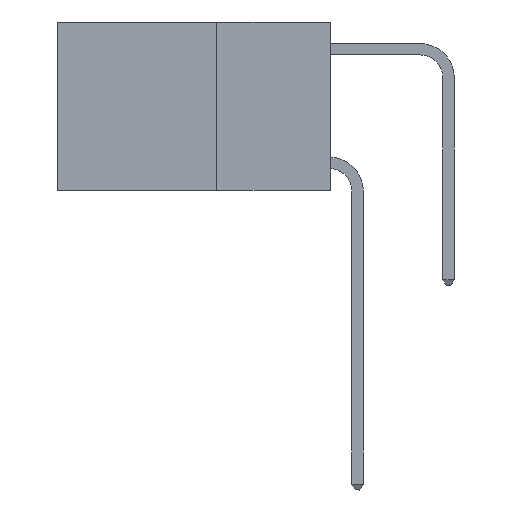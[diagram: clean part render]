
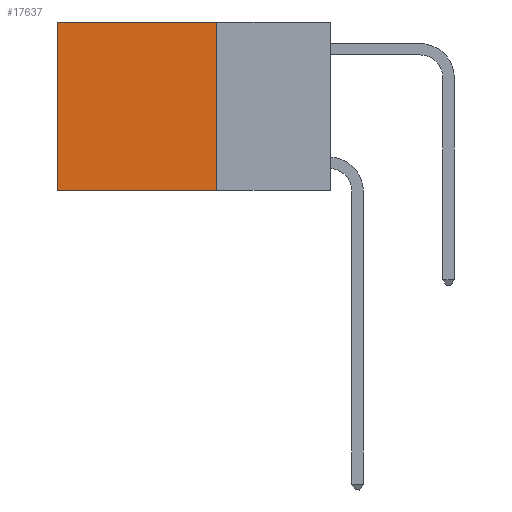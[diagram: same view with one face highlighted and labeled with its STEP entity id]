
A CAD part, left-side view. The second image highlights one B-rep face of the part: STEP entity #17637.
In plain terms, the highlighted planar face has unit normal (-1, 0, 0).
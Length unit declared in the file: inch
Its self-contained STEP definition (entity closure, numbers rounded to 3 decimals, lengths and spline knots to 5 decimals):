
#320 = ORIENTED_EDGE ( 'NONE', *, *, #20586, .F. ) ;
#1253 = CARTESIAN_POINT ( 'NONE',  ( 0.2625, 0.6, 0. ) ) ;
#2351 = AXIS2_PLACEMENT_3D ( 'NONE', #25943, #19576, #7491 ) ;
#5475 = ORIENTED_EDGE ( 'NONE', *, *, #19314, .T. ) ;
#5598 = ORIENTED_EDGE ( 'NONE', *, *, #20037, .F. ) ;
#6199 = VECTOR ( 'NONE', #19068, 39.37008 ) ;
#6403 = CARTESIAN_POINT ( 'NONE',  ( 0.2625, 0.25, 0. ) ) ;
#6913 = VERTEX_POINT ( 'NONE', #6403 ) ;
#7078 = VERTEX_POINT ( 'NONE', #18467 ) ;
#7491 = DIRECTION ( 'NONE',  ( 0., 0., -1. ) ) ;
#7664 = DIRECTION ( 'NONE',  ( 0., 0., -1. ) ) ;
#8567 = DIRECTION ( 'NONE',  ( 0., 1., 0. ) ) ;
#11240 = LINE ( 'NONE', #18738, #12729 ) ;
#11598 = PLANE ( 'NONE',  #2351 ) ;
#12692 = VECTOR ( 'NONE', #8567, 39.37008 ) ;
#12729 = VECTOR ( 'NONE', #25596, 39.37008 ) ;
#13668 = CARTESIAN_POINT ( 'NONE',  ( 0.2625, 0.25, -0.37 ) ) ;
#17259 = EDGE_LOOP ( 'NONE', ( #25081, #5598, #320, #5475 ) ) ;
#17589 = LINE ( 'NONE', #1253, #25044 ) ;
#17637 = ADVANCED_FACE ( 'NONE', ( #19714 ), #11598, .F. ) ;
#18467 = CARTESIAN_POINT ( 'NONE',  ( 0.2625, 0.6, -0.37 ) ) ;
#18738 = CARTESIAN_POINT ( 'NONE',  ( 0.2625, 0.25, -0.37 ) ) ;
#19068 = DIRECTION ( 'NONE',  ( 0., 0., -1. ) ) ;
#19282 = CARTESIAN_POINT ( 'NONE',  ( 0.2625, 0.25, 0. ) ) ;
#19314 = EDGE_CURVE ( 'NONE', #6913, #21622, #21300, .T. ) ;
#19334 = LINE ( 'NONE', #21101, #6199 ) ;
#19576 = DIRECTION ( 'NONE',  ( 1., 0., 0. ) ) ;
#19714 = FACE_OUTER_BOUND ( 'NONE', #17259, .T. ) ;
#20037 = EDGE_CURVE ( 'NONE', #26081, #7078, #11240, .T. ) ;
#20586 = EDGE_CURVE ( 'NONE', #6913, #26081, #19334, .T. ) ;
#21101 = CARTESIAN_POINT ( 'NONE',  ( 0.2625, 0.25, 0. ) ) ;
#21300 = LINE ( 'NONE', #19282, #12692 ) ;
#21622 = VERTEX_POINT ( 'NONE', #26560 ) ;
#25044 = VECTOR ( 'NONE', #7664, 39.37008 ) ;
#25081 = ORIENTED_EDGE ( 'NONE', *, *, #26074, .T. ) ;
#25596 = DIRECTION ( 'NONE',  ( 0., 1., 0. ) ) ;
#25943 = CARTESIAN_POINT ( 'NONE',  ( 0.2625, 0.25, 0. ) ) ;
#26074 = EDGE_CURVE ( 'NONE', #21622, #7078, #17589, .T. ) ;
#26081 = VERTEX_POINT ( 'NONE', #13668 ) ;
#26560 = CARTESIAN_POINT ( 'NONE',  ( 0.2625, 0.6, 0. ) ) ;
